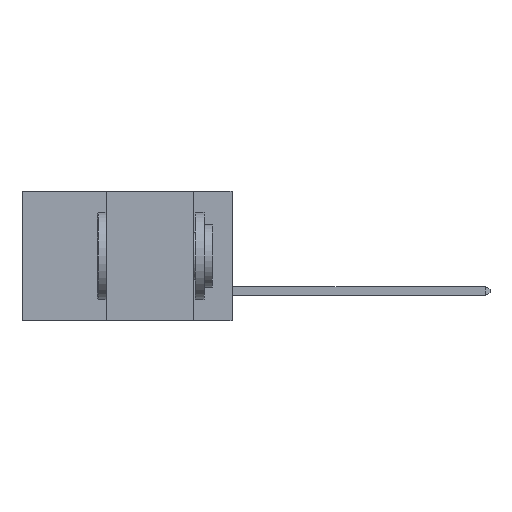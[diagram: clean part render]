
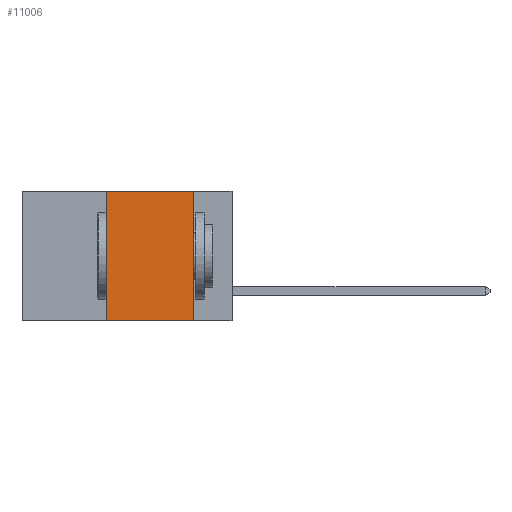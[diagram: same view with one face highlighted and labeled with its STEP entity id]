
A CAD part, left-side view. The second image highlights one B-rep face of the part: STEP entity #11006.
In plain terms, the highlighted planar face has unit normal (-1, 0, 0).
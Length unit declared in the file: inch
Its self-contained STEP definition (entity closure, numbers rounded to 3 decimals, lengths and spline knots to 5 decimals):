
#360 = VERTEX_POINT ( 'NONE', #11540 ) ;
#1055 = VERTEX_POINT ( 'NONE', #5583 ) ;
#1806 = EDGE_CURVE ( 'NONE', #360, #15607, #3392, .T. ) ;
#2646 = DIRECTION ( 'NONE',  ( 1., 0., 0. ) ) ;
#2872 = EDGE_LOOP ( 'NONE', ( #9199, #14463, #10812, #13660 ) ) ;
#3392 = LINE ( 'NONE', #6306, #13449 ) ;
#3875 = LINE ( 'NONE', #11417, #13955 ) ;
#4623 = CARTESIAN_POINT ( 'NONE',  ( 0., 0.36, 0. ) ) ;
#5556 = LINE ( 'NONE', #4623, #8694 ) ;
#5583 = CARTESIAN_POINT ( 'NONE',  ( 0., 0.11, -0.37 ) ) ;
#6264 = DIRECTION ( 'NONE',  ( 0., -1., 0. ) ) ;
#6306 = CARTESIAN_POINT ( 'NONE',  ( 0., 0.6, 0. ) ) ;
#6822 = EDGE_CURVE ( 'NONE', #8193, #360, #5556, .T. ) ;
#7487 = CARTESIAN_POINT ( 'NONE',  ( 0., 0.11, 0. ) ) ;
#7624 = DIRECTION ( 'NONE',  ( 0., -1., 0. ) ) ;
#8150 = LINE ( 'NONE', #13462, #11557 ) ;
#8193 = VERTEX_POINT ( 'NONE', #11633 ) ;
#8694 = VECTOR ( 'NONE', #16233, 39.37008 ) ;
#9199 = ORIENTED_EDGE ( 'NONE', *, *, #16538, .F. ) ;
#10472 = CARTESIAN_POINT ( 'NONE',  ( 0., 0.6, 0. ) ) ;
#10812 = ORIENTED_EDGE ( 'NONE', *, *, #6822, .F. ) ;
#11006 = ADVANCED_FACE ( 'NONE', ( #12001 ), #14320, .F. ) ;
#11417 = CARTESIAN_POINT ( 'NONE',  ( 0., 0.6, -0.37 ) ) ;
#11540 = CARTESIAN_POINT ( 'NONE',  ( 0., 0.36, 0. ) ) ;
#11557 = VECTOR ( 'NONE', #14670, 39.37008 ) ;
#11633 = CARTESIAN_POINT ( 'NONE',  ( 0., 0.36, -0.37 ) ) ;
#11780 = DIRECTION ( 'NONE',  ( 0., 0., -1. ) ) ;
#12001 = FACE_OUTER_BOUND ( 'NONE', #2872, .T. ) ;
#13449 = VECTOR ( 'NONE', #6264, 39.37008 ) ;
#13462 = CARTESIAN_POINT ( 'NONE',  ( 0., 0.11, 0. ) ) ;
#13660 = ORIENTED_EDGE ( 'NONE', *, *, #14942, .T. ) ;
#13955 = VECTOR ( 'NONE', #7624, 39.37008 ) ;
#14320 = PLANE ( 'NONE',  #16466 ) ;
#14463 = ORIENTED_EDGE ( 'NONE', *, *, #1806, .F. ) ;
#14670 = DIRECTION ( 'NONE',  ( 0., 0., -1. ) ) ;
#14942 = EDGE_CURVE ( 'NONE', #8193, #1055, #3875, .T. ) ;
#15607 = VERTEX_POINT ( 'NONE', #7487 ) ;
#16233 = DIRECTION ( 'NONE',  ( 0., 0., 1. ) ) ;
#16466 = AXIS2_PLACEMENT_3D ( 'NONE', #10472, #2646, #11780 ) ;
#16538 = EDGE_CURVE ( 'NONE', #15607, #1055, #8150, .T. ) ;
